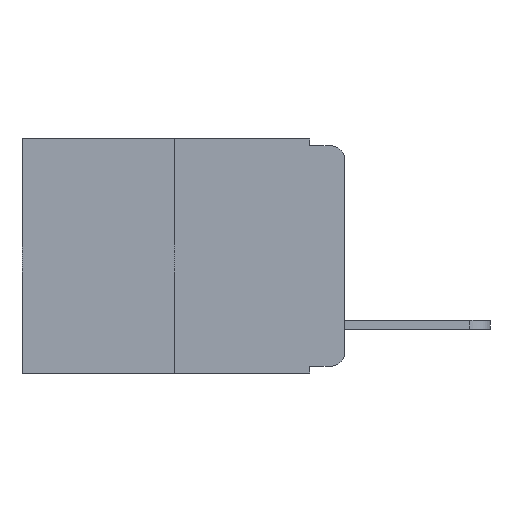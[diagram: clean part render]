
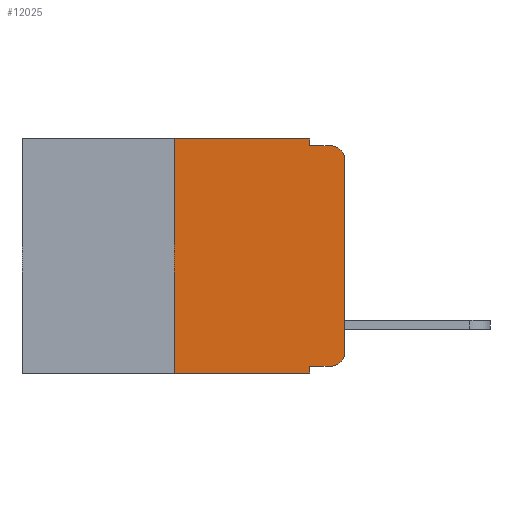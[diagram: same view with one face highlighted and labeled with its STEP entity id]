
A CAD part, left-side view. The second image highlights one B-rep face of the part: STEP entity #12025.
In plain terms, the highlighted planar face has unit normal (-1, 0, 0).
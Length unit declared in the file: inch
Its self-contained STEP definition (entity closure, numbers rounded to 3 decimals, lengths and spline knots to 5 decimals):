
#102 = CARTESIAN_POINT ( 'NONE',  ( 0., 0.25, 0. ) ) ;
#450 = DIRECTION ( 'NONE',  ( 0., 0., -1. ) ) ;
#1149 = CARTESIAN_POINT ( 'NONE',  ( 0., 0.051, -0.333 ) ) ;
#1296 = CARTESIAN_POINT ( 'NONE',  ( 0., 0.051, 0. ) ) ;
#1326 = EDGE_LOOP ( 'NONE', ( #10322, #1337, #8556, #4762, #17196, #4777, #19892, #13031, #4163, #8726 ) ) ;
#1337 = ORIENTED_EDGE ( 'NONE', *, *, #15012, .T. ) ;
#1347 = VERTEX_POINT ( 'NONE', #9158 ) ;
#1626 = AXIS2_PLACEMENT_3D ( 'NONE', #12651, #2927, #14212 ) ;
#1883 = VECTOR ( 'NONE', #9624, 39.37008 ) ;
#2307 = VERTEX_POINT ( 'NONE', #13153 ) ;
#2550 = CARTESIAN_POINT ( 'NONE',  ( 0., 0., -0.03 ) ) ;
#2770 = VECTOR ( 'NONE', #8214, 39.37008 ) ;
#2927 = DIRECTION ( 'NONE',  ( -1., 0., 0. ) ) ;
#2950 = VERTEX_POINT ( 'NONE', #13667 ) ;
#3050 = VECTOR ( 'NONE', #6342, 39.37008 ) ;
#3261 = DIRECTION ( 'NONE',  ( -1., 0., 0. ) ) ;
#3328 = DIRECTION ( 'NONE',  ( 0., -1., 0. ) ) ;
#3995 = VERTEX_POINT ( 'NONE', #5066 ) ;
#4130 = CARTESIAN_POINT ( 'NONE',  ( 0., 0.473, 0. ) ) ;
#4163 = ORIENTED_EDGE ( 'NONE', *, *, #15326, .T. ) ;
#4762 = ORIENTED_EDGE ( 'NONE', *, *, #15185, .F. ) ;
#4777 = ORIENTED_EDGE ( 'NONE', *, *, #15271, .F. ) ;
#4906 = LINE ( 'NONE', #15935, #16353 ) ;
#5066 = CARTESIAN_POINT ( 'NONE',  ( 0., 0.02, -0.333 ) ) ;
#5313 = LINE ( 'NONE', #10089, #17128 ) ;
#5749 = VERTEX_POINT ( 'NONE', #19378 ) ;
#6342 = DIRECTION ( 'NONE',  ( 0., 0., 1. ) ) ;
#6481 = CARTESIAN_POINT ( 'NONE',  ( 0., 0.051, 0. ) ) ;
#7128 = LINE ( 'NONE', #6481, #10737 ) ;
#7854 = VERTEX_POINT ( 'NONE', #19131 ) ;
#8078 = VECTOR ( 'NONE', #11950, 39.37008 ) ;
#8214 = DIRECTION ( 'NONE',  ( 0., -1., 0. ) ) ;
#8556 = ORIENTED_EDGE ( 'NONE', *, *, #15068, .F. ) ;
#8726 = ORIENTED_EDGE ( 'NONE', *, *, #15388, .T. ) ;
#9158 = CARTESIAN_POINT ( 'NONE',  ( 0., 0.051, -0.01 ) ) ;
#9624 = DIRECTION ( 'NONE',  ( 0., -1., 0. ) ) ;
#9681 = CARTESIAN_POINT ( 'NONE',  ( 0., 0.051, -0.01 ) ) ;
#10089 = CARTESIAN_POINT ( 'NONE',  ( 0., 0.051, 0. ) ) ;
#10322 = ORIENTED_EDGE ( 'NONE', *, *, #14892, .T. ) ;
#10411 = CARTESIAN_POINT ( 'NONE',  ( 0., 0.473, 0. ) ) ;
#10628 = DIRECTION ( 'NONE',  ( 1., 0., 0. ) ) ;
#10737 = VECTOR ( 'NONE', #19862, 39.37008 ) ;
#11616 = DIRECTION ( 'NONE',  ( 0., 0., -1. ) ) ;
#11950 = DIRECTION ( 'NONE',  ( 0., -1., 0. ) ) ;
#11964 = LINE ( 'NONE', #9681, #2770 ) ;
#12025 = ADVANCED_FACE ( 'NONE', ( #16651 ), #19395, .F. ) ;
#12507 = EDGE_CURVE ( 'NONE', #17599, #13408, #19400, .T. ) ;
#12651 = CARTESIAN_POINT ( 'NONE',  ( 0., 0.02, -0.03 ) ) ;
#12656 = VERTEX_POINT ( 'NONE', #2550 ) ;
#12939 = CARTESIAN_POINT ( 'NONE',  ( 0., 0.02, -0.313 ) ) ;
#12945 = CIRCLE ( 'NONE', #1626, 0.02 ) ;
#13031 = ORIENTED_EDGE ( 'NONE', *, *, #15308, .F. ) ;
#13153 = CARTESIAN_POINT ( 'NONE',  ( 0., 0.25, -0.343 ) ) ;
#13351 = AXIS2_PLACEMENT_3D ( 'NONE', #12939, #3261, #14457 ) ;
#13408 = VERTEX_POINT ( 'NONE', #1296 ) ;
#13457 = EDGE_CURVE ( 'NONE', #2307, #2950, #4906, .T. ) ;
#13667 = CARTESIAN_POINT ( 'NONE',  ( 0., 0.051, -0.343 ) ) ;
#13777 = DIRECTION ( 'NONE',  ( 0., 0., 1. ) ) ;
#14212 = DIRECTION ( 'NONE',  ( 0., 0., -1. ) ) ;
#14378 = VECTOR ( 'NONE', #13777, 39.37008 ) ;
#14457 = DIRECTION ( 'NONE',  ( 0., 0., -1. ) ) ;
#14892 = EDGE_CURVE ( 'NONE', #7854, #12656, #19029, .T. ) ;
#15012 = EDGE_CURVE ( 'NONE', #12656, #16073, #12945, .T. ) ;
#15068 = EDGE_CURVE ( 'NONE', #1347, #16073, #11964, .T. ) ;
#15185 = EDGE_CURVE ( 'NONE', #13408, #1347, #5313, .T. ) ;
#15271 = EDGE_CURVE ( 'NONE', #2307, #17599, #15739, .T. ) ;
#15308 = EDGE_CURVE ( 'NONE', #5749, #2950, #7128, .T. ) ;
#15326 = EDGE_CURVE ( 'NONE', #5749, #3995, #19010, .T. ) ;
#15388 = EDGE_CURVE ( 'NONE', #3995, #7854, #17338, .T. ) ;
#15739 = LINE ( 'NONE', #17044, #3050 ) ;
#15935 = CARTESIAN_POINT ( 'NONE',  ( 0., 0.473, -0.343 ) ) ;
#16073 = VERTEX_POINT ( 'NONE', #16457 ) ;
#16353 = VECTOR ( 'NONE', #3328, 39.37008 ) ;
#16457 = CARTESIAN_POINT ( 'NONE',  ( 0., 0.02, -0.01 ) ) ;
#16651 = FACE_OUTER_BOUND ( 'NONE', #1326, .T. ) ;
#17044 = CARTESIAN_POINT ( 'NONE',  ( 0., 0.25, 0. ) ) ;
#17128 = VECTOR ( 'NONE', #11616, 39.37008 ) ;
#17196 = ORIENTED_EDGE ( 'NONE', *, *, #12507, .F. ) ;
#17338 = CIRCLE ( 'NONE', #13351, 0.02 ) ;
#17599 = VERTEX_POINT ( 'NONE', #102 ) ;
#19010 = LINE ( 'NONE', #1149, #1883 ) ;
#19029 = LINE ( 'NONE', #19401, #14378 ) ;
#19131 = CARTESIAN_POINT ( 'NONE',  ( 0., 0., -0.313 ) ) ;
#19378 = CARTESIAN_POINT ( 'NONE',  ( 0., 0.051, -0.333 ) ) ;
#19395 = PLANE ( 'NONE',  #20380 ) ;
#19400 = LINE ( 'NONE', #10411, #8078 ) ;
#19401 = CARTESIAN_POINT ( 'NONE',  ( 0., 0., 0. ) ) ;
#19862 = DIRECTION ( 'NONE',  ( 0., 0., -1. ) ) ;
#19892 = ORIENTED_EDGE ( 'NONE', *, *, #13457, .T. ) ;
#20380 = AXIS2_PLACEMENT_3D ( 'NONE', #4130, #10628, #450 ) ;
